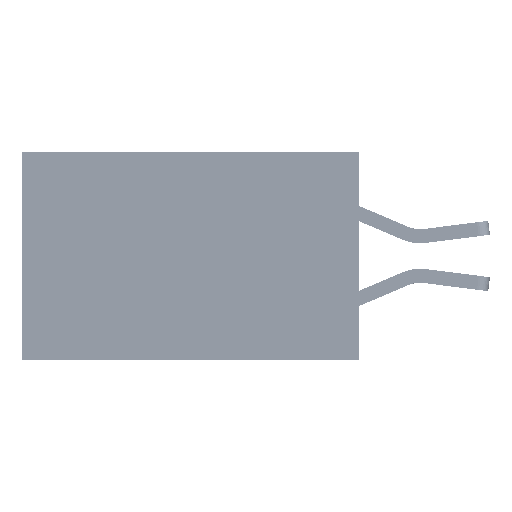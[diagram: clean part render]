
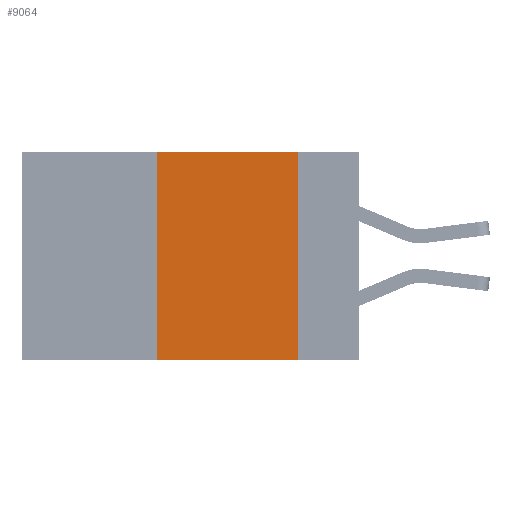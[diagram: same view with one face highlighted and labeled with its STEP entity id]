
A CAD part, left-side view. The second image highlights one B-rep face of the part: STEP entity #9064.
In plain terms, the highlighted planar face has unit normal (-1, 0, 0).
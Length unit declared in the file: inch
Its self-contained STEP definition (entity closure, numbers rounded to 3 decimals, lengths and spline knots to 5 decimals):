
#355 = DIRECTION ( 'NONE',  ( 0., -1., 0. ) ) ;
#359 = EDGE_CURVE ( 'NONE', #3240, #26145, #20689, .T. ) ;
#755 = PLANE ( 'NONE',  #25851 ) ;
#1619 = ORIENTED_EDGE ( 'NONE', *, *, #13514, .T. ) ;
#1653 = CARTESIAN_POINT ( 'NONE',  ( 0., 0.36, 0. ) ) ;
#3108 = VECTOR ( 'NONE', #22931, 39.37008 ) ;
#3240 = VERTEX_POINT ( 'NONE', #6741 ) ;
#6089 = LINE ( 'NONE', #20064, #10470 ) ;
#6741 = CARTESIAN_POINT ( 'NONE',  ( 0., 0.36, -0.37 ) ) ;
#8051 = CARTESIAN_POINT ( 'NONE',  ( 0., 0.36, 0. ) ) ;
#8305 = LINE ( 'NONE', #25134, #13684 ) ;
#9064 = ADVANCED_FACE ( 'NONE', ( #17982 ), #755, .F. ) ;
#10470 = VECTOR ( 'NONE', #13404, 39.37008 ) ;
#11170 = EDGE_CURVE ( 'NONE', #39845, #33085, #6089, .T. ) ;
#13191 = DIRECTION ( 'NONE',  ( 0., 0., -1. ) ) ;
#13404 = DIRECTION ( 'NONE',  ( 0., 0., -1. ) ) ;
#13514 = EDGE_CURVE ( 'NONE', #3240, #33085, #15913, .T. ) ;
#13684 = VECTOR ( 'NONE', #35022, 39.37008 ) ;
#13990 = VECTOR ( 'NONE', #355, 39.37008 ) ;
#15446 = ORIENTED_EDGE ( 'NONE', *, *, #359, .F. ) ;
#15905 = CARTESIAN_POINT ( 'NONE',  ( 0., 0.6, -0.37 ) ) ;
#15913 = LINE ( 'NONE', #15905, #13990 ) ;
#16777 = ORIENTED_EDGE ( 'NONE', *, *, #11170, .F. ) ;
#17982 = FACE_OUTER_BOUND ( 'NONE', #33418, .T. ) ;
#20064 = CARTESIAN_POINT ( 'NONE',  ( 0., 0.11, 0. ) ) ;
#20689 = LINE ( 'NONE', #1653, #3108 ) ;
#22931 = DIRECTION ( 'NONE',  ( 0., 0., 1. ) ) ;
#25134 = CARTESIAN_POINT ( 'NONE',  ( 0., 0.6, 0. ) ) ;
#25851 = AXIS2_PLACEMENT_3D ( 'NONE', #31863, #38208, #13191 ) ;
#26145 = VERTEX_POINT ( 'NONE', #8051 ) ;
#27041 = CARTESIAN_POINT ( 'NONE',  ( 0., 0.11, 0. ) ) ;
#31863 = CARTESIAN_POINT ( 'NONE',  ( 0., 0.6, 0. ) ) ;
#32806 = CARTESIAN_POINT ( 'NONE',  ( 0., 0.11, -0.37 ) ) ;
#33085 = VERTEX_POINT ( 'NONE', #32806 ) ;
#33418 = EDGE_LOOP ( 'NONE', ( #16777, #36001, #15446, #1619 ) ) ;
#33770 = EDGE_CURVE ( 'NONE', #26145, #39845, #8305, .T. ) ;
#35022 = DIRECTION ( 'NONE',  ( 0., -1., 0. ) ) ;
#36001 = ORIENTED_EDGE ( 'NONE', *, *, #33770, .F. ) ;
#38208 = DIRECTION ( 'NONE',  ( 1., 0., 0. ) ) ;
#39845 = VERTEX_POINT ( 'NONE', #27041 ) ;
